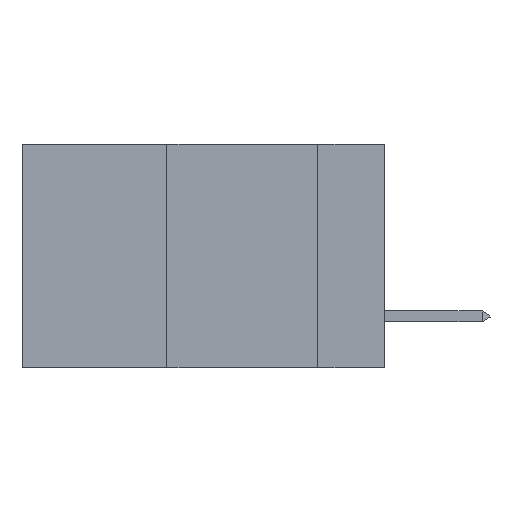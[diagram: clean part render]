
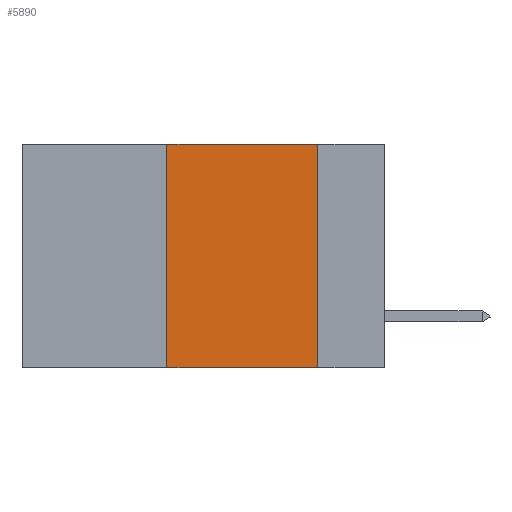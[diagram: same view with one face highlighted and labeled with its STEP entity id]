
A CAD part, left-side view. The second image highlights one B-rep face of the part: STEP entity #5890.
In plain terms, the highlighted planar face has unit normal (-1, 0, 0).
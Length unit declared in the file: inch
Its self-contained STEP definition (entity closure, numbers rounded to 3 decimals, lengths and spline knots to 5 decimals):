
#251 = DIRECTION ( 'NONE',  ( 0., -1., 0. ) ) ;
#509 = DIRECTION ( 'NONE',  ( 1., 0., 0. ) ) ;
#688 = LINE ( 'NONE', #18326, #23936 ) ;
#777 = ORIENTED_EDGE ( 'NONE', *, *, #9643, .F. ) ;
#3083 = ORIENTED_EDGE ( 'NONE', *, *, #13794, .T. ) ;
#3422 = DIRECTION ( 'NONE',  ( 0., 0., 1. ) ) ;
#3805 = EDGE_LOOP ( 'NONE', ( #777, #20446, #17657, #3083 ) ) ;
#4320 = PLANE ( 'NONE',  #7759 ) ;
#5273 = VECTOR ( 'NONE', #3422, 39.37008 ) ;
#5890 = ADVANCED_FACE ( 'NONE', ( #19436 ), #4320, .F. ) ;
#7759 = AXIS2_PLACEMENT_3D ( 'NONE', #8427, #509, #22262 ) ;
#8427 = CARTESIAN_POINT ( 'NONE',  ( 0., 0.6, 0. ) ) ;
#9292 = DIRECTION ( 'NONE',  ( 0., 0., -1. ) ) ;
#9616 = LINE ( 'NONE', #15342, #5273 ) ;
#9643 = EDGE_CURVE ( 'NONE', #13604, #17656, #20742, .T. ) ;
#9670 = EDGE_CURVE ( 'NONE', #19170, #18303, #9616, .T. ) ;
#10984 = CARTESIAN_POINT ( 'NONE',  ( 0., 0.36, 0. ) ) ;
#11472 = VECTOR ( 'NONE', #9292, 39.37008 ) ;
#13519 = VECTOR ( 'NONE', #251, 39.37008 ) ;
#13604 = VERTEX_POINT ( 'NONE', #23263 ) ;
#13794 = EDGE_CURVE ( 'NONE', #19170, #17656, #25256, .T. ) ;
#14503 = DIRECTION ( 'NONE',  ( 0., -1., 0. ) ) ;
#15179 = CARTESIAN_POINT ( 'NONE',  ( 0., 0.11, 0. ) ) ;
#15342 = CARTESIAN_POINT ( 'NONE',  ( 0., 0.36, 0. ) ) ;
#16128 = CARTESIAN_POINT ( 'NONE',  ( 0., 0.36, -0.37 ) ) ;
#17188 = CARTESIAN_POINT ( 'NONE',  ( 0., 0.6, -0.37 ) ) ;
#17656 = VERTEX_POINT ( 'NONE', #21745 ) ;
#17657 = ORIENTED_EDGE ( 'NONE', *, *, #9670, .F. ) ;
#17705 = EDGE_CURVE ( 'NONE', #18303, #13604, #688, .T. ) ;
#18303 = VERTEX_POINT ( 'NONE', #10984 ) ;
#18326 = CARTESIAN_POINT ( 'NONE',  ( 0., 0.6, 0. ) ) ;
#19170 = VERTEX_POINT ( 'NONE', #16128 ) ;
#19436 = FACE_OUTER_BOUND ( 'NONE', #3805, .T. ) ;
#20446 = ORIENTED_EDGE ( 'NONE', *, *, #17705, .F. ) ;
#20742 = LINE ( 'NONE', #15179, #11472 ) ;
#21745 = CARTESIAN_POINT ( 'NONE',  ( 0., 0.11, -0.37 ) ) ;
#22262 = DIRECTION ( 'NONE',  ( 0., 0., -1. ) ) ;
#23263 = CARTESIAN_POINT ( 'NONE',  ( 0., 0.11, 0. ) ) ;
#23936 = VECTOR ( 'NONE', #14503, 39.37008 ) ;
#25256 = LINE ( 'NONE', #17188, #13519 ) ;
